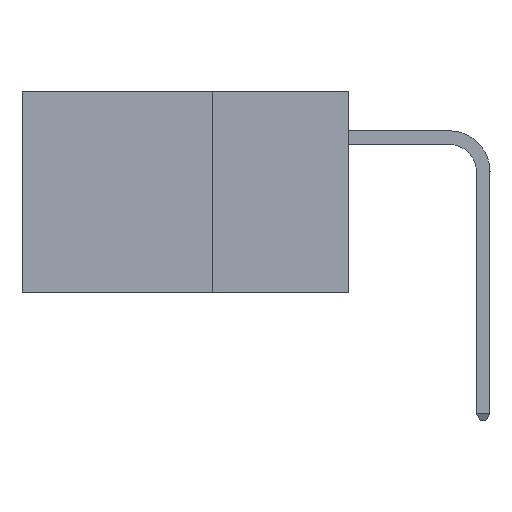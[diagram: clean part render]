
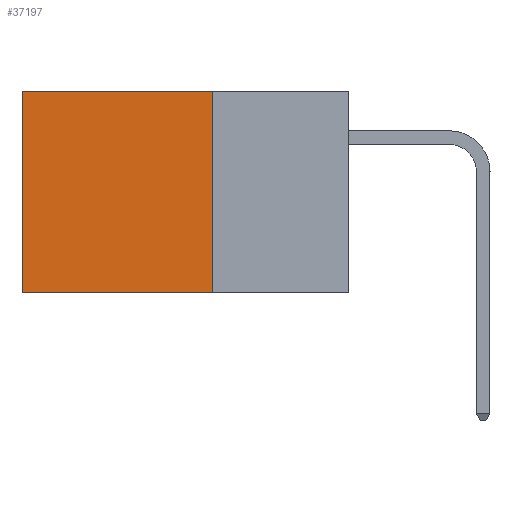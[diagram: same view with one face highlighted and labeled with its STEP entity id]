
A CAD part, left-side view. The second image highlights one B-rep face of the part: STEP entity #37197.
In plain terms, the highlighted planar face has unit normal (-1, 0, 0).
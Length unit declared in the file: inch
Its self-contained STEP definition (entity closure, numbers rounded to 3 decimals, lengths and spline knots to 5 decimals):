
#394 = VECTOR ( 'NONE', #19135, 39.37008 ) ;
#561 = EDGE_CURVE ( 'NONE', #33884, #10063, #8062, .T. ) ;
#1335 = LINE ( 'NONE', #33854, #394 ) ;
#4013 = ORIENTED_EDGE ( 'NONE', *, *, #20682, .F. ) ;
#8062 = LINE ( 'NONE', #9785, #15055 ) ;
#8965 = VERTEX_POINT ( 'NONE', #9164 ) ;
#9164 = CARTESIAN_POINT ( 'NONE',  ( 0.2875, 0.25, -0.37 ) ) ;
#9759 = VECTOR ( 'NONE', #9986, 39.37008 ) ;
#9785 = CARTESIAN_POINT ( 'NONE',  ( 0.2875, 0.25, 0. ) ) ;
#9986 = DIRECTION ( 'NONE',  ( 0., 0., -1. ) ) ;
#10063 = VERTEX_POINT ( 'NONE', #11163 ) ;
#11163 = CARTESIAN_POINT ( 'NONE',  ( 0.2875, 0.6, 0. ) ) ;
#11232 = ORIENTED_EDGE ( 'NONE', *, *, #561, .T. ) ;
#13524 = DIRECTION ( 'NONE',  ( 0., 0., -1. ) ) ;
#15055 = VECTOR ( 'NONE', #15904, 39.37008 ) ;
#15904 = DIRECTION ( 'NONE',  ( 0., 1., 0. ) ) ;
#16875 = EDGE_CURVE ( 'NONE', #8965, #36488, #32079, .T. ) ;
#17178 = ORIENTED_EDGE ( 'NONE', *, *, #17301, .T. ) ;
#17301 = EDGE_CURVE ( 'NONE', #10063, #36488, #1335, .T. ) ;
#19135 = DIRECTION ( 'NONE',  ( 0., 0., -1. ) ) ;
#19358 = PLANE ( 'NONE',  #25717 ) ;
#20682 = EDGE_CURVE ( 'NONE', #33884, #8965, #24604, .T. ) ;
#21642 = ORIENTED_EDGE ( 'NONE', *, *, #16875, .F. ) ;
#22336 = CARTESIAN_POINT ( 'NONE',  ( 0.2875, 0.25, 0. ) ) ;
#23935 = EDGE_LOOP ( 'NONE', ( #17178, #21642, #4013, #11232 ) ) ;
#24181 = VECTOR ( 'NONE', #37758, 39.37008 ) ;
#24345 = CARTESIAN_POINT ( 'NONE',  ( 0.2875, 0.6, -0.37 ) ) ;
#24604 = LINE ( 'NONE', #24771, #9759 ) ;
#24771 = CARTESIAN_POINT ( 'NONE',  ( 0.2875, 0.25, 0. ) ) ;
#25717 = AXIS2_PLACEMENT_3D ( 'NONE', #22336, #31301, #13524 ) ;
#28114 = CARTESIAN_POINT ( 'NONE',  ( 0.2875, 0.25, 0. ) ) ;
#28868 = CARTESIAN_POINT ( 'NONE',  ( 0.2875, 0.25, -0.37 ) ) ;
#31301 = DIRECTION ( 'NONE',  ( 1., 0., 0. ) ) ;
#32079 = LINE ( 'NONE', #28868, #24181 ) ;
#32844 = FACE_OUTER_BOUND ( 'NONE', #23935, .T. ) ;
#33854 = CARTESIAN_POINT ( 'NONE',  ( 0.2875, 0.6, 0. ) ) ;
#33884 = VERTEX_POINT ( 'NONE', #28114 ) ;
#36488 = VERTEX_POINT ( 'NONE', #24345 ) ;
#37197 = ADVANCED_FACE ( 'NONE', ( #32844 ), #19358, .F. ) ;
#37758 = DIRECTION ( 'NONE',  ( 0., 1., 0. ) ) ;
